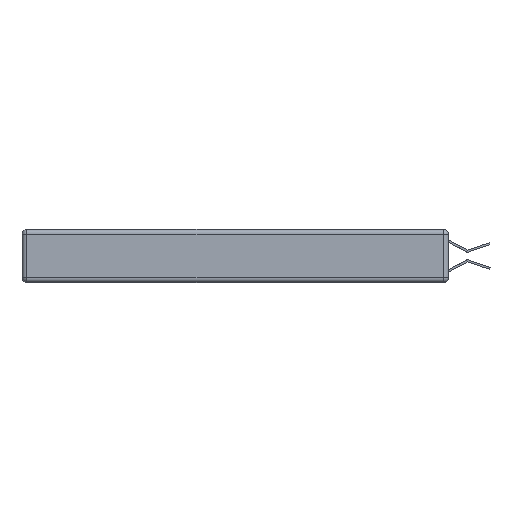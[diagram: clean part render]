
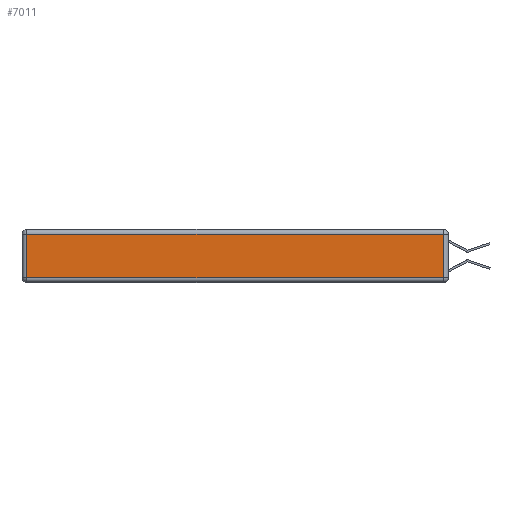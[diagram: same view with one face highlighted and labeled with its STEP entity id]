
A CAD part, left-side view. The second image highlights one B-rep face of the part: STEP entity #7011.
In plain terms, the highlighted planar face has unit normal (-1, 0, 0).
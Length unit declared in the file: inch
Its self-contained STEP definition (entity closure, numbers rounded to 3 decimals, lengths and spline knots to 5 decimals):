
#783 = VECTOR ( 'NONE', #9519, 39.37008 ) ;
#1028 = LINE ( 'NONE', #4968, #6167 ) ;
#1614 = CARTESIAN_POINT ( 'NONE',  ( 0., 2.75, -0.03 ) ) ;
#2265 = EDGE_CURVE ( 'NONE', #4625, #2764, #11262, .T. ) ;
#2764 = VERTEX_POINT ( 'NONE', #10398 ) ;
#2870 = DIRECTION ( 'NONE',  ( 0., 0., 1. ) ) ;
#3704 = EDGE_CURVE ( 'NONE', #2764, #9802, #6453, .T. ) ;
#4006 = ORIENTED_EDGE ( 'NONE', *, *, #12740, .T. ) ;
#4306 = CARTESIAN_POINT ( 'NONE',  ( 0., 0.03, -0.343 ) ) ;
#4451 = ORIENTED_EDGE ( 'NONE', *, *, #2265, .T. ) ;
#4625 = VERTEX_POINT ( 'NONE', #6164 ) ;
#4968 = CARTESIAN_POINT ( 'NONE',  ( 0., 0., -0.313 ) ) ;
#5078 = DIRECTION ( 'NONE',  ( -1., 0., 0. ) ) ;
#5114 = EDGE_LOOP ( 'NONE', ( #7992, #4451, #9516, #4006 ) ) ;
#5395 = CARTESIAN_POINT ( 'NONE',  ( 0., 2.72, -0.343 ) ) ;
#6164 = CARTESIAN_POINT ( 'NONE',  ( 0., 0.03, -0.313 ) ) ;
#6167 = VECTOR ( 'NONE', #10470, 39.37008 ) ;
#6453 = LINE ( 'NONE', #1614, #783 ) ;
#6688 = VERTEX_POINT ( 'NONE', #13770 ) ;
#7011 = ADVANCED_FACE ( 'NONE', ( #9624 ), #12910, .T. ) ;
#7154 = AXIS2_PLACEMENT_3D ( 'NONE', #11812, #5078, #2870 ) ;
#7582 = DIRECTION ( 'NONE',  ( 0., 0., 1. ) ) ;
#7992 = ORIENTED_EDGE ( 'NONE', *, *, #10486, .T. ) ;
#8378 = LINE ( 'NONE', #5395, #10541 ) ;
#8763 = VECTOR ( 'NONE', #7582, 39.37008 ) ;
#9516 = ORIENTED_EDGE ( 'NONE', *, *, #3704, .T. ) ;
#9519 = DIRECTION ( 'NONE',  ( 0., 1., 0. ) ) ;
#9624 = FACE_OUTER_BOUND ( 'NONE', #5114, .T. ) ;
#9802 = VERTEX_POINT ( 'NONE', #13769 ) ;
#10398 = CARTESIAN_POINT ( 'NONE',  ( 0., 0.03, -0.03 ) ) ;
#10470 = DIRECTION ( 'NONE',  ( 0., -1., 0. ) ) ;
#10486 = EDGE_CURVE ( 'NONE', #6688, #4625, #1028, .T. ) ;
#10541 = VECTOR ( 'NONE', #13098, 39.37008 ) ;
#11262 = LINE ( 'NONE', #4306, #8763 ) ;
#11812 = CARTESIAN_POINT ( 'NONE',  ( 0., 0., -0.343 ) ) ;
#12740 = EDGE_CURVE ( 'NONE', #9802, #6688, #8378, .T. ) ;
#12910 = PLANE ( 'NONE',  #7154 ) ;
#13098 = DIRECTION ( 'NONE',  ( 0., 0., -1. ) ) ;
#13769 = CARTESIAN_POINT ( 'NONE',  ( 0., 2.72, -0.03 ) ) ;
#13770 = CARTESIAN_POINT ( 'NONE',  ( 0., 2.72, -0.313 ) ) ;
